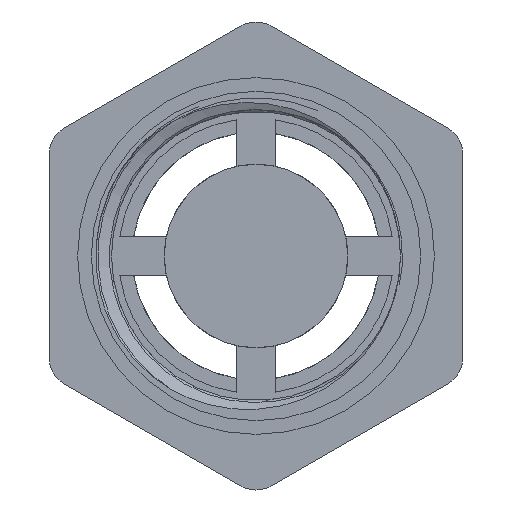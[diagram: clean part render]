
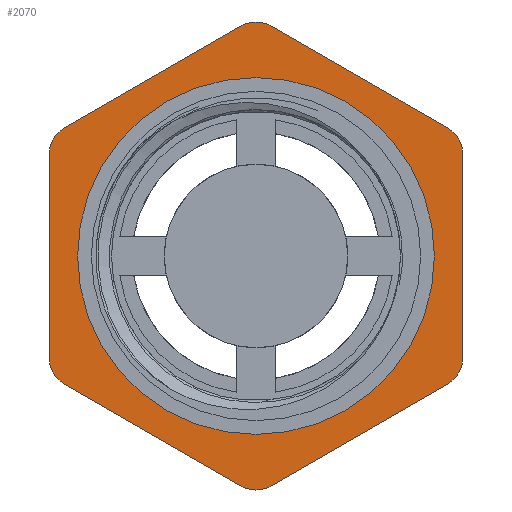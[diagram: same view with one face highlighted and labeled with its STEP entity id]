
A CAD part, front view. The second image highlights one B-rep face of the part: STEP entity #2070.
In plain terms, the highlighted planar face has unit normal (0, -1, 0).
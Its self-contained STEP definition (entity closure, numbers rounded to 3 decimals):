
#35=FACE_BOUND('',#278,.T.);
#68=PLANE('',#2286);
#166=FACE_OUTER_BOUND('',#277,.T.);
#277=EDGE_LOOP('',(#1715,#1716,#1717,#1718,#1719,#1720,#1721,#1722,#1723,
#1724,#1725,#1726));
#278=EDGE_LOOP('',(#1727));
#374=CIRCLE('',#2253,2.);
#382=CIRCLE('',#2266,2.);
#383=CIRCLE('',#2268,2.);
#384=CIRCLE('',#2271,2.);
#385=CIRCLE('',#2273,2.);
#386=CIRCLE('',#2276,2.);
#389=CIRCLE('',#2283,11.672);
#553=LINE('',#3932,#687);
#606=LINE('',#4289,#740);
#607=LINE('',#4291,#741);
#610=LINE('',#4306,#744);
#611=LINE('',#4307,#745);
#612=LINE('',#4308,#746);
#687=VECTOR('',#2519,10.);
#740=VECTOR('',#2756,10.);
#741=VECTOR('',#2759,10.);
#744=VECTOR('',#2778,10.);
#745=VECTOR('',#2779,10.);
#746=VECTOR('',#2780,10.);
#886=VERTEX_POINT('',#3929);
#887=VERTEX_POINT('',#3931);
#937=VERTEX_POINT('',#4239);
#941=VERTEX_POINT('',#4257);
#942=VERTEX_POINT('',#4258);
#943=VERTEX_POINT('',#4263);
#944=VERTEX_POINT('',#4264);
#945=VERTEX_POINT('',#4271);
#946=VERTEX_POINT('',#4272);
#947=VERTEX_POINT('',#4277);
#948=VERTEX_POINT('',#4278);
#949=VERTEX_POINT('',#4285);
#952=VERTEX_POINT('',#4299);
#1128=EDGE_CURVE('',#887,#886,#553,.T.);
#1217=EDGE_CURVE('',#887,#937,#374,.T.);
#1226=EDGE_CURVE('',#941,#942,#382,.T.);
#1229=EDGE_CURVE('',#943,#944,#383,.T.);
#1233=EDGE_CURVE('',#945,#946,#384,.T.);
#1236=EDGE_CURVE('',#947,#948,#385,.T.);
#1240=EDGE_CURVE('',#949,#886,#386,.T.);
#1242=EDGE_CURVE('',#941,#946,#606,.T.);
#1243=EDGE_CURVE('',#945,#937,#607,.T.);
#1247=EDGE_CURVE('',#952,#952,#389,.T.);
#1250=EDGE_CURVE('',#949,#948,#610,.T.);
#1251=EDGE_CURVE('',#947,#944,#611,.T.);
#1252=EDGE_CURVE('',#943,#942,#612,.T.);
#1715=ORIENTED_EDGE('',*,*,#1226,.F.);
#1716=ORIENTED_EDGE('',*,*,#1242,.T.);
#1717=ORIENTED_EDGE('',*,*,#1233,.F.);
#1718=ORIENTED_EDGE('',*,*,#1243,.T.);
#1719=ORIENTED_EDGE('',*,*,#1217,.F.);
#1720=ORIENTED_EDGE('',*,*,#1128,.T.);
#1721=ORIENTED_EDGE('',*,*,#1240,.F.);
#1722=ORIENTED_EDGE('',*,*,#1250,.T.);
#1723=ORIENTED_EDGE('',*,*,#1236,.F.);
#1724=ORIENTED_EDGE('',*,*,#1251,.T.);
#1725=ORIENTED_EDGE('',*,*,#1229,.F.);
#1726=ORIENTED_EDGE('',*,*,#1252,.T.);
#1727=ORIENTED_EDGE('',*,*,#1247,.T.);
#2070=ADVANCED_FACE('',(#166,#35),#68,.T.);
#2253=AXIS2_PLACEMENT_3D('',#4240,#2694,#2695);
#2266=AXIS2_PLACEMENT_3D('',#4259,#2721,#2722);
#2268=AXIS2_PLACEMENT_3D('',#4265,#2727,#2728);
#2271=AXIS2_PLACEMENT_3D('',#4273,#2736,#2737);
#2273=AXIS2_PLACEMENT_3D('',#4279,#2742,#2743);
#2276=AXIS2_PLACEMENT_3D('',#4286,#2751,#2752);
#2283=AXIS2_PLACEMENT_3D('',#4300,#2769,#2770);
#2286=AXIS2_PLACEMENT_3D('',#4305,#2776,#2777);
#2519=DIRECTION('',(0.,0.,1.));
#2694=DIRECTION('center_axis',(0.,1.,0.));
#2695=DIRECTION('ref_axis',(0.866,0.,-0.5));
#2721=DIRECTION('center_axis',(0.,1.,0.));
#2722=DIRECTION('ref_axis',(-0.866,0.,-0.5));
#2727=DIRECTION('center_axis',(0.,1.,0.));
#2728=DIRECTION('ref_axis',(-0.866,0.,0.5));
#2736=DIRECTION('center_axis',(0.,1.,0.));
#2737=DIRECTION('ref_axis',(0.,0.,-1.));
#2742=DIRECTION('center_axis',(0.,1.,0.));
#2743=DIRECTION('ref_axis',(0.,0.,1.));
#2751=DIRECTION('center_axis',(0.,1.,0.));
#2752=DIRECTION('ref_axis',(0.866,0.,0.5));
#2756=DIRECTION('',(0.866,0.,-0.5));
#2759=DIRECTION('',(0.866,0.,0.5));
#2769=DIRECTION('center_axis',(0.,1.,0.));
#2770=DIRECTION('ref_axis',(-1.,0.,0.));
#2776=DIRECTION('center_axis',(0.,-1.,0.));
#2777=DIRECTION('ref_axis',(0.,0.,-1.));
#2778=DIRECTION('',(-0.866,0.,0.5));
#2779=DIRECTION('',(-0.866,0.,-0.5));
#2780=DIRECTION('',(0.,0.,-1.));
#3929=CARTESIAN_POINT('',(13.524,-25.4,6.653));
#3931=CARTESIAN_POINT('',(13.524,-25.4,-6.653));
#3932=CARTESIAN_POINT('',(13.524,-25.4,-7.808));
#4239=CARTESIAN_POINT('',(12.524,-25.4,-8.385));
#4240=CARTESIAN_POINT('Origin',(11.524,-25.4,-6.653));
#4257=CARTESIAN_POINT('',(-12.524,-25.4,-8.385));
#4258=CARTESIAN_POINT('',(-13.524,-25.4,-6.653));
#4259=CARTESIAN_POINT('Origin',(-11.524,-25.4,-6.653));
#4263=CARTESIAN_POINT('',(-13.524,-25.4,6.653));
#4264=CARTESIAN_POINT('',(-12.524,-25.4,8.385));
#4265=CARTESIAN_POINT('Origin',(-11.524,-25.4,6.653));
#4271=CARTESIAN_POINT('',(1.,-25.4,-15.038));
#4272=CARTESIAN_POINT('',(-1.,-25.4,-15.038));
#4273=CARTESIAN_POINT('Origin',(0.,-25.4,-13.306));
#4277=CARTESIAN_POINT('',(-1.,-25.4,15.038));
#4278=CARTESIAN_POINT('',(1.,-25.4,15.038));
#4279=CARTESIAN_POINT('Origin',(0.,-25.4,13.306));
#4285=CARTESIAN_POINT('',(12.524,-25.4,8.385));
#4286=CARTESIAN_POINT('Origin',(11.524,-25.4,6.653));
#4289=CARTESIAN_POINT('',(-13.524,-25.4,-7.808));
#4291=CARTESIAN_POINT('',(0.,-25.4,-15.616));
#4299=CARTESIAN_POINT('',(11.672,-25.4,0.));
#4300=CARTESIAN_POINT('Origin',(0.,-25.4,0.));
#4305=CARTESIAN_POINT('Origin',(0.,-25.4,0.));
#4306=CARTESIAN_POINT('',(13.524,-25.4,7.808));
#4307=CARTESIAN_POINT('',(0.,-25.4,15.616));
#4308=CARTESIAN_POINT('',(-13.524,-25.4,7.808));
